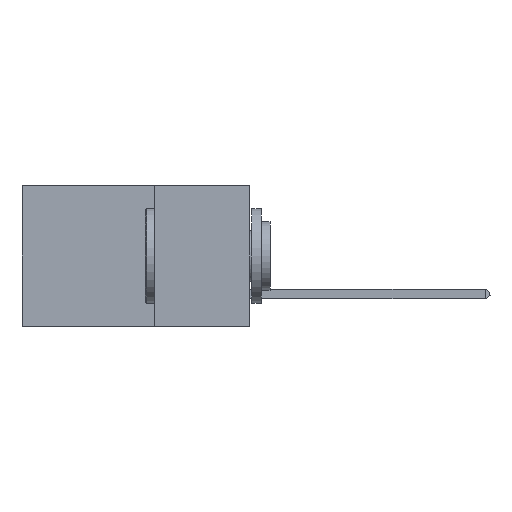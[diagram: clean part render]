
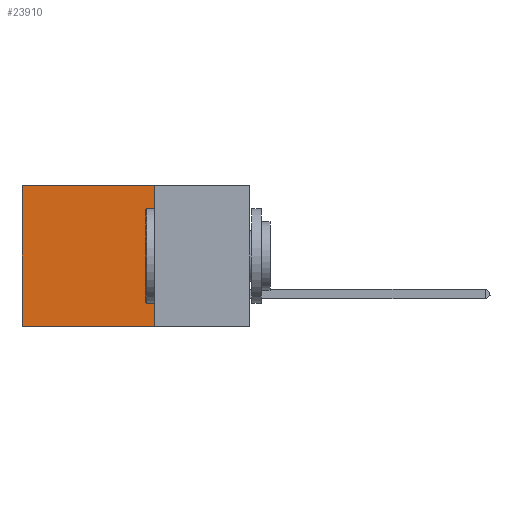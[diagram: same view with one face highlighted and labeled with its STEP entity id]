
A CAD part, left-side view. The second image highlights one B-rep face of the part: STEP entity #23910.
In plain terms, the highlighted planar face has unit normal (-1, 0, 0).
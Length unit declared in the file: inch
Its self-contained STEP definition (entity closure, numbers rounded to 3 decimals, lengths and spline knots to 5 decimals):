
#1313 = VERTEX_POINT ( 'NONE', #9874 ) ;
#2992 = CARTESIAN_POINT ( 'NONE',  ( 0.2875, 0.25, -0.37 ) ) ;
#3617 = CARTESIAN_POINT ( 'NONE',  ( 0.2875, 0.25, 0. ) ) ;
#3779 = EDGE_LOOP ( 'NONE', ( #44397, #7491, #40847, #21160 ) ) ;
#6023 = CARTESIAN_POINT ( 'NONE',  ( 0.2875, 0.6, 0. ) ) ;
#6936 = LINE ( 'NONE', #2992, #13013 ) ;
#7491 = ORIENTED_EDGE ( 'NONE', *, *, #16045, .F. ) ;
#9874 = CARTESIAN_POINT ( 'NONE',  ( 0.2875, 0.6, 0. ) ) ;
#12044 = VERTEX_POINT ( 'NONE', #29264 ) ;
#12057 = CARTESIAN_POINT ( 'NONE',  ( 0.2875, 0.25, 0. ) ) ;
#13013 = VECTOR ( 'NONE', #37979, 39.37008 ) ;
#13517 = LINE ( 'NONE', #3617, #29076 ) ;
#14467 = CARTESIAN_POINT ( 'NONE',  ( 0.2875, 0.25, 0. ) ) ;
#16045 = EDGE_CURVE ( 'NONE', #12044, #27753, #6936, .T. ) ;
#18796 = EDGE_CURVE ( 'NONE', #37781, #12044, #44188, .T. ) ;
#20341 = CARTESIAN_POINT ( 'NONE',  ( 0.2875, 0.6, -0.37 ) ) ;
#20405 = PLANE ( 'NONE',  #32204 ) ;
#21018 = DIRECTION ( 'NONE',  ( 1., 0., 0. ) ) ;
#21160 = ORIENTED_EDGE ( 'NONE', *, *, #27256, .T. ) ;
#22073 = VECTOR ( 'NONE', #38807, 39.37008 ) ;
#23910 = ADVANCED_FACE ( 'NONE', ( #30747 ), #20405, .F. ) ;
#25084 = CARTESIAN_POINT ( 'NONE',  ( 0.2875, 0.25, 0. ) ) ;
#27256 = EDGE_CURVE ( 'NONE', #37781, #1313, #13517, .T. ) ;
#27753 = VERTEX_POINT ( 'NONE', #20341 ) ;
#28441 = DIRECTION ( 'NONE',  ( 0., 0., -1. ) ) ;
#28738 = VECTOR ( 'NONE', #34352, 39.37008 ) ;
#29076 = VECTOR ( 'NONE', #45871, 39.37008 ) ;
#29264 = CARTESIAN_POINT ( 'NONE',  ( 0.2875, 0.25, -0.37 ) ) ;
#30747 = FACE_OUTER_BOUND ( 'NONE', #3779, .T. ) ;
#32204 = AXIS2_PLACEMENT_3D ( 'NONE', #14467, #21018, #28441 ) ;
#34352 = DIRECTION ( 'NONE',  ( 0., 0., -1. ) ) ;
#37311 = EDGE_CURVE ( 'NONE', #1313, #27753, #44747, .T. ) ;
#37781 = VERTEX_POINT ( 'NONE', #12057 ) ;
#37979 = DIRECTION ( 'NONE',  ( 0., 1., 0. ) ) ;
#38807 = DIRECTION ( 'NONE',  ( 0., 0., -1. ) ) ;
#40847 = ORIENTED_EDGE ( 'NONE', *, *, #18796, .F. ) ;
#44188 = LINE ( 'NONE', #25084, #22073 ) ;
#44397 = ORIENTED_EDGE ( 'NONE', *, *, #37311, .T. ) ;
#44747 = LINE ( 'NONE', #6023, #28738 ) ;
#45871 = DIRECTION ( 'NONE',  ( 0., 1., 0. ) ) ;
